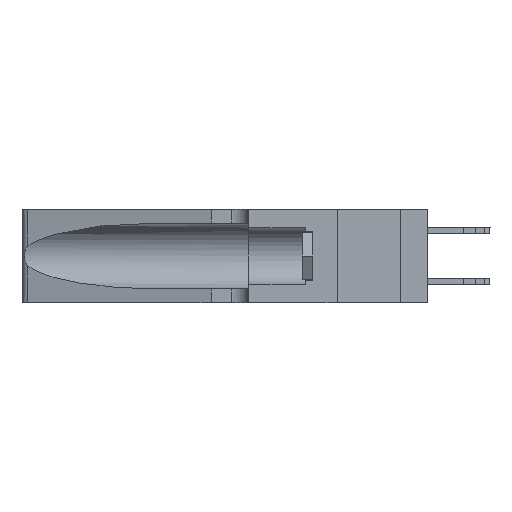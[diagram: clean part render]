
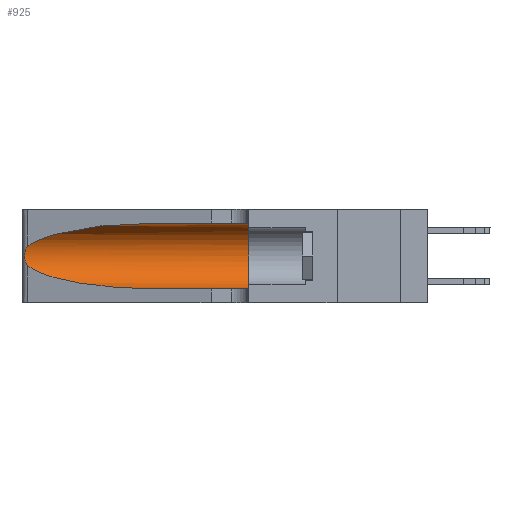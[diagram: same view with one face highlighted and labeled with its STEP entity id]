
A CAD part, left-side view. The second image highlights one B-rep face of the part: STEP entity #925.
In plain terms, the highlighted cylindrical face has radius 3.308 mm (diameter 6.617 mm), a partial arc.
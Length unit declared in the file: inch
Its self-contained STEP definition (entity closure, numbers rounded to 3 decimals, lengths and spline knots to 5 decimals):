
#925 = ADVANCED_FACE ( 'NONE', ( #19255 ), #14635, .F. ) ;
#2130 = AXIS2_PLACEMENT_3D ( 'NONE', #2712, #5510, #2578 ) ;
#2493 = ORIENTED_EDGE ( 'NONE', *, *, #14359, .T. ) ;
#2578 = DIRECTION ( 'NONE',  ( 0., 0., -1. ) ) ;
#2712 = CARTESIAN_POINT ( 'NONE',  ( 0.1305, 1.61858, 0.185 ) ) ;
#2780 = CARTESIAN_POINT ( 'NONE',  ( 0.25789, 1.23486, 0.15765 ) ) ;
#2888 = CARTESIAN_POINT ( 'NONE',  ( 0.25555, 1.22994, 0.2215 ) ) ;
#3118 = CARTESIAN_POINT ( 'NONE',  ( 0.26075, 1.23896, 0.19203 ) ) ;
#3950 = CARTESIAN_POINT ( 'NONE',  ( 0.25487, 1.22718, 0.22369 ) ) ;
#4487 = VERTEX_POINT ( 'NONE', #12690 ) ;
#4990 =( BOUNDED_CURVE ( )  B_SPLINE_CURVE ( 3, ( #31063, #23317, #12555, #31560 ),
 .UNSPECIFIED., .F., .F. ) 
 B_SPLINE_CURVE_WITH_KNOTS ( ( 4, 4 ),
 ( 3.44316, 4.71239 ),
 .UNSPECIFIED. ) 
 CURVE ( )  GEOMETRIC_REPRESENTATION_ITEM ( )  RATIONAL_B_SPLINE_CURVE ( ( 1., 0.87, 0.87, 1. ) ) 
 REPRESENTATION_ITEM ( '' )  );
#5510 = DIRECTION ( 'NONE',  ( 0., -1., 0. ) ) ;
#5829 = CARTESIAN_POINT ( 'NONE',  ( 0.25555, 1.22993, 0.14849 ) ) ;
#6921 = VERTEX_POINT ( 'NONE', #27720 ) ;
#6984 = VERTEX_POINT ( 'NONE', #9603 ) ;
#7696 = ORIENTED_EDGE ( 'NONE', *, *, #28585, .T. ) ;
#7890 = EDGE_CURVE ( 'NONE', #6921, #15182, #18856, .T. ) ;
#8415 = CARTESIAN_POINT ( 'NONE',  ( 0.25639, 1.23186, 0.15144 ) ) ;
#8667 =( BOUNDED_CURVE ( )  B_SPLINE_CURVE ( 3, ( #19431, #20247, #11996, #3950 ),
 .UNSPECIFIED., .F., .T. ) 
 B_SPLINE_CURVE_WITH_KNOTS ( ( 4, 4 ),
 ( 1.5708, 2.84003 ),
 .UNSPECIFIED. ) 
 CURVE ( )  GEOMETRIC_REPRESENTATION_ITEM ( )  RATIONAL_B_SPLINE_CURVE ( ( 1., 0.87, 0.87, 1. ) ) 
 REPRESENTATION_ITEM ( '' )  );
#9390 = CARTESIAN_POINT ( 'NONE',  ( 0.25487, 1.22718, 0.14631 ) ) ;
#9603 = CARTESIAN_POINT ( 'NONE',  ( 0.25487, 1.22718, 0.22369 ) ) ;
#10492 = DIRECTION ( 'NONE',  ( 0., -1., 0. ) ) ;
#10888 = VECTOR ( 'NONE', #29391, 39.37008 ) ;
#10937 = CARTESIAN_POINT ( 'NONE',  ( 0.26018, 1.23835, 0.19895 ) ) ;
#11996 = CARTESIAN_POINT ( 'NONE',  ( 0.2373, 1.15595, 0.28018 ) ) ;
#12529 = DIRECTION ( 'NONE',  ( 0., 1., 0. ) ) ;
#12555 = CARTESIAN_POINT ( 'NONE',  ( 0.18966, 0.96281, 0.05475 ) ) ;
#12690 = CARTESIAN_POINT ( 'NONE',  ( 0.1305, 0.72297, 0.31525 ) ) ;
#13428 = CARTESIAN_POINT ( 'NONE',  ( 0.25787, 1.23484, 0.2124 ) ) ;
#13830 = EDGE_CURVE ( 'NONE', #4487, #32914, #18083, .T. ) ;
#14359 = EDGE_CURVE ( 'NONE', #30934, #6921, #4990, .T. ) ;
#14635 = CYLINDRICAL_SURFACE ( 'NONE', #2130, 0.13025 ) ;
#15182 = VERTEX_POINT ( 'NONE', #27292 ) ;
#16458 = CARTESIAN_POINT ( 'NONE',  ( 0.25854, 1.2359, 0.20912 ) ) ;
#17988 = EDGE_CURVE ( 'NONE', #32914, #15182, #26986, .T. ) ;
#18083 = LINE ( 'NONE', #26044, #10888 ) ;
#18097 = CARTESIAN_POINT ( 'NONE',  ( 0.1305, 0.35, 0.185 ) ) ;
#18199 = DIRECTION ( 'NONE',  ( 0., 0., 1. ) ) ;
#18856 = LINE ( 'NONE', #26438, #26453 ) ;
#18969 = CARTESIAN_POINT ( 'NONE',  ( 0.25487, 1.22718, 0.14631 ) ) ;
#19255 = FACE_OUTER_BOUND ( 'NONE', #30162, .T. ) ;
#19309 = CARTESIAN_POINT ( 'NONE',  ( 0.25639, 1.23184, 0.21858 ) ) ;
#19431 = CARTESIAN_POINT ( 'NONE',  ( 0.1305, 0.72297, 0.31525 ) ) ;
#20247 = CARTESIAN_POINT ( 'NONE',  ( 0.18966, 0.96281, 0.31525 ) ) ;
#21577 = CARTESIAN_POINT ( 'NONE',  ( 0.25856, 1.23593, 0.16098 ) ) ;
#23317 = CARTESIAN_POINT ( 'NONE',  ( 0.2373, 1.15595, 0.08982 ) ) ;
#24163 = ORIENTED_EDGE ( 'NONE', *, *, #17988, .F. ) ;
#24500 = AXIS2_PLACEMENT_3D ( 'NONE', #18097, #12529, #18199 ) ;
#24633 = CARTESIAN_POINT ( 'NONE',  ( 0.26075, 1.23896, 0.178 ) ) ;
#24862 = ORIENTED_EDGE ( 'NONE', *, *, #7890, .T. ) ;
#25669 = CARTESIAN_POINT ( 'NONE',  ( 0.1305, 0.35, 0.31525 ) ) ;
#26044 = CARTESIAN_POINT ( 'NONE',  ( 0.1305, 1.61858, 0.31525 ) ) ;
#26438 = CARTESIAN_POINT ( 'NONE',  ( 0.1305, 1.61858, 0.05475 ) ) ;
#26453 = VECTOR ( 'NONE', #10492, 39.37008 ) ;
#26986 = CIRCLE ( 'NONE', #24500, 0.13025 ) ;
#27052 = ORIENTED_EDGE ( 'NONE', *, *, #30918, .T. ) ;
#27292 = CARTESIAN_POINT ( 'NONE',  ( 0.1305, 0.35, 0.05475 ) ) ;
#27720 = CARTESIAN_POINT ( 'NONE',  ( 0.1305, 0.72297, 0.05475 ) ) ;
#28585 = EDGE_CURVE ( 'NONE', #6984, #30934, #30184, .T. ) ;
#29083 = CARTESIAN_POINT ( 'NONE',  ( 0.25487, 1.22718, 0.22369 ) ) ;
#29391 = DIRECTION ( 'NONE',  ( 0., -1., 0. ) ) ;
#30110 = CARTESIAN_POINT ( 'NONE',  ( 0.26017, 1.23833, 0.17102 ) ) ;
#30162 = EDGE_LOOP ( 'NONE', ( #27052, #7696, #2493, #24862, #24163, #32253 ) ) ;
#30184 = B_SPLINE_CURVE_WITH_KNOTS ( 'NONE', 3,
 ( #29083, #2888, #19309, #13428, #16458, #10937, #3118, #24633, #30110, #21577, #2780, #8415, #5829, #18969 ),
 .UNSPECIFIED., .F., .F.,
 ( 4, 2, 2, 2, 2, 2, 4 ),
 ( 0., 0.00027, 0.00053, 0.00107, 0.0016, 0.00187, 0.00214 ),
 .UNSPECIFIED. ) ;
#30918 = EDGE_CURVE ( 'NONE', #4487, #6984, #8667, .T. ) ;
#30934 = VERTEX_POINT ( 'NONE', #9390 ) ;
#31063 = CARTESIAN_POINT ( 'NONE',  ( 0.25487, 1.22718, 0.14631 ) ) ;
#31560 = CARTESIAN_POINT ( 'NONE',  ( 0.1305, 0.72297, 0.05475 ) ) ;
#32253 = ORIENTED_EDGE ( 'NONE', *, *, #13830, .F. ) ;
#32914 = VERTEX_POINT ( 'NONE', #25669 ) ;
